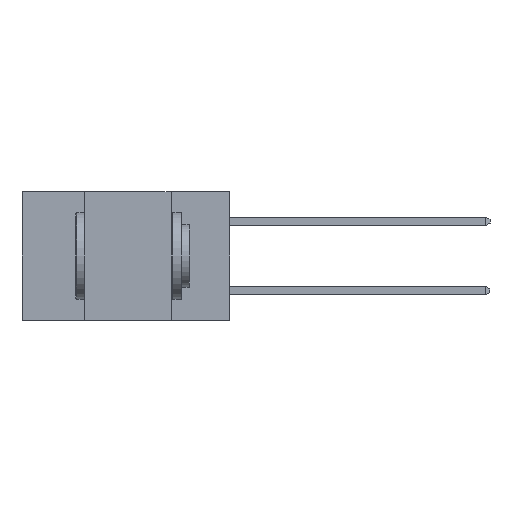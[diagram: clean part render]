
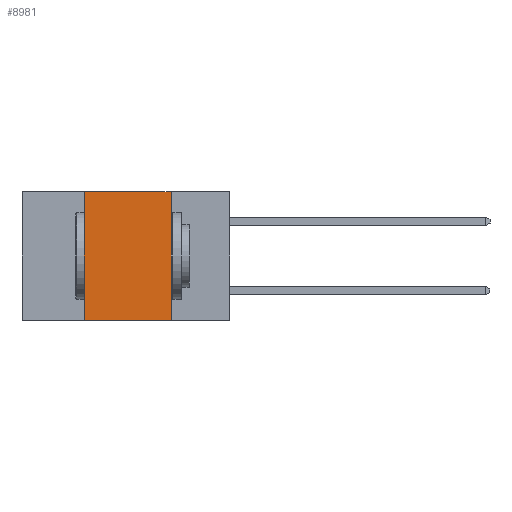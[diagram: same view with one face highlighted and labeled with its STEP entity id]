
A CAD part, left-side view. The second image highlights one B-rep face of the part: STEP entity #8981.
In plain terms, the highlighted planar face has unit normal (-1, 0, 0).
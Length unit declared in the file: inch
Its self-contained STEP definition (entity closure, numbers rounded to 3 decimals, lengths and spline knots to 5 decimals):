
#1283 = CARTESIAN_POINT ( 'NONE',  ( 0., 0.6, -0.37 ) ) ;
#1442 = EDGE_CURVE ( 'NONE', #25070, #13170, #4495, .T. ) ;
#1789 = LINE ( 'NONE', #14246, #21177 ) ;
#2977 = VECTOR ( 'NONE', #23867, 39.37008 ) ;
#3731 = AXIS2_PLACEMENT_3D ( 'NONE', #20773, #8649, #25652 ) ;
#3763 = PLANE ( 'NONE',  #3731 ) ;
#4495 = LINE ( 'NONE', #24839, #2977 ) ;
#5943 = VECTOR ( 'NONE', #30492, 39.37008 ) ;
#6597 = EDGE_CURVE ( 'NONE', #13170, #31302, #11762, .T. ) ;
#8649 = DIRECTION ( 'NONE',  ( 1., 0., 0. ) ) ;
#8981 = ADVANCED_FACE ( 'NONE', ( #13418 ), #3763, .F. ) ;
#9493 = CARTESIAN_POINT ( 'NONE',  ( 0., 0.42, -0.37 ) ) ;
#11762 = LINE ( 'NONE', #20711, #30421 ) ;
#12375 = LINE ( 'NONE', #1283, #5943 ) ;
#13170 = VERTEX_POINT ( 'NONE', #24507 ) ;
#13418 = FACE_OUTER_BOUND ( 'NONE', #19301, .T. ) ;
#14181 = EDGE_CURVE ( 'NONE', #19397, #25070, #1789, .T. ) ;
#14246 = CARTESIAN_POINT ( 'NONE',  ( 0., 0.42, 0. ) ) ;
#14683 = EDGE_CURVE ( 'NONE', #19397, #31302, #12375, .T. ) ;
#17234 = ORIENTED_EDGE ( 'NONE', *, *, #14181, .F. ) ;
#17348 = CARTESIAN_POINT ( 'NONE',  ( 0., 0.17, -0.37 ) ) ;
#19301 = EDGE_LOOP ( 'NONE', ( #21035, #26330, #17234, #24752 ) ) ;
#19397 = VERTEX_POINT ( 'NONE', #9493 ) ;
#20711 = CARTESIAN_POINT ( 'NONE',  ( 0., 0.17, 0. ) ) ;
#20773 = CARTESIAN_POINT ( 'NONE',  ( 0., 0.6, 0. ) ) ;
#21035 = ORIENTED_EDGE ( 'NONE', *, *, #6597, .F. ) ;
#21177 = VECTOR ( 'NONE', #31256, 39.37008 ) ;
#23867 = DIRECTION ( 'NONE',  ( 0., -1., 0. ) ) ;
#24507 = CARTESIAN_POINT ( 'NONE',  ( 0., 0.17, 0. ) ) ;
#24752 = ORIENTED_EDGE ( 'NONE', *, *, #14683, .T. ) ;
#24839 = CARTESIAN_POINT ( 'NONE',  ( 0., 0.6, 0. ) ) ;
#25070 = VERTEX_POINT ( 'NONE', #27347 ) ;
#25652 = DIRECTION ( 'NONE',  ( 0., 0., -1. ) ) ;
#26330 = ORIENTED_EDGE ( 'NONE', *, *, #1442, .F. ) ;
#27347 = CARTESIAN_POINT ( 'NONE',  ( 0., 0.42, 0. ) ) ;
#28010 = DIRECTION ( 'NONE',  ( 0., 0., -1. ) ) ;
#30421 = VECTOR ( 'NONE', #28010, 39.37008 ) ;
#30492 = DIRECTION ( 'NONE',  ( 0., -1., 0. ) ) ;
#31256 = DIRECTION ( 'NONE',  ( 0., 0., 1. ) ) ;
#31302 = VERTEX_POINT ( 'NONE', #17348 ) ;
